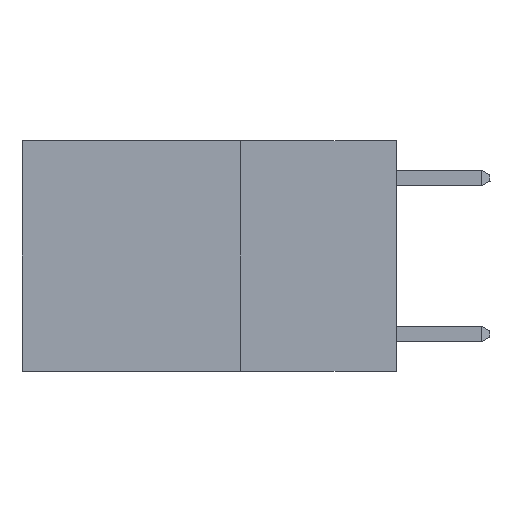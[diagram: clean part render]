
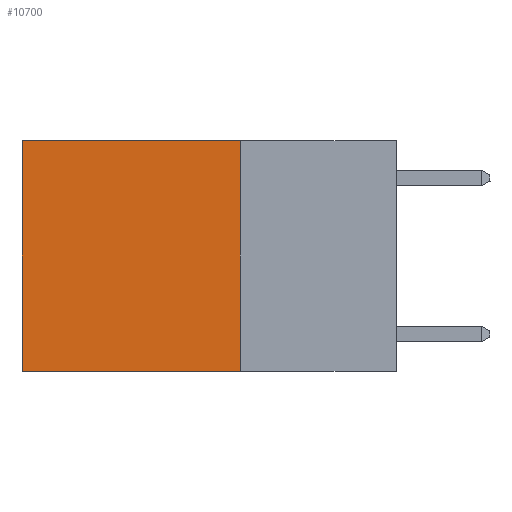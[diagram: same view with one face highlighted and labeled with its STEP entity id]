
A CAD part, left-side view. The second image highlights one B-rep face of the part: STEP entity #10700.
In plain terms, the highlighted planar face has unit normal (-1, 0, 0).
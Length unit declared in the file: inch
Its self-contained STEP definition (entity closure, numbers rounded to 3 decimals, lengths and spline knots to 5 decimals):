
#1501 = VERTEX_POINT ( 'NONE', #17438 ) ;
#1979 = EDGE_CURVE ( 'NONE', #24790, #1501, #23777, .T. ) ;
#2228 = DIRECTION ( 'NONE',  ( 0., 0., -1. ) ) ;
#2391 = VECTOR ( 'NONE', #21699, 39.37008 ) ;
#3250 = ORIENTED_EDGE ( 'NONE', *, *, #13745, .F. ) ;
#4246 = LINE ( 'NONE', #12738, #13555 ) ;
#4757 = CARTESIAN_POINT ( 'NONE',  ( 0.2625, 0.25, -0.37 ) ) ;
#6575 = DIRECTION ( 'NONE',  ( 0., 1., 0. ) ) ;
#9055 = DIRECTION ( 'NONE',  ( 0., 0., -1. ) ) ;
#9156 = VECTOR ( 'NONE', #6575, 39.37008 ) ;
#10002 = EDGE_LOOP ( 'NONE', ( #15845, #26331, #3250, #17077 ) ) ;
#10683 = VECTOR ( 'NONE', #9055, 39.37008 ) ;
#10700 = ADVANCED_FACE ( 'NONE', ( #14855 ), #15138, .F. ) ;
#11227 = CARTESIAN_POINT ( 'NONE',  ( 0.2625, 0.25, -0.37 ) ) ;
#12738 = CARTESIAN_POINT ( 'NONE',  ( 0.2625, 0.25, 0. ) ) ;
#13242 = LINE ( 'NONE', #23913, #10683 ) ;
#13253 = CARTESIAN_POINT ( 'NONE',  ( 0.2625, 0.6, 0. ) ) ;
#13555 = VECTOR ( 'NONE', #25208, 39.37008 ) ;
#13745 = EDGE_CURVE ( 'NONE', #18843, #26649, #13242, .T. ) ;
#14855 = FACE_OUTER_BOUND ( 'NONE', #10002, .T. ) ;
#15138 = PLANE ( 'NONE',  #23408 ) ;
#15565 = CARTESIAN_POINT ( 'NONE',  ( 0.2625, 0.25, 0. ) ) ;
#15845 = ORIENTED_EDGE ( 'NONE', *, *, #1979, .T. ) ;
#17077 = ORIENTED_EDGE ( 'NONE', *, *, #21356, .T. ) ;
#17438 = CARTESIAN_POINT ( 'NONE',  ( 0.2625, 0.6, -0.37 ) ) ;
#18843 = VERTEX_POINT ( 'NONE', #15565 ) ;
#20287 = CARTESIAN_POINT ( 'NONE',  ( 0.2625, 0.6, 0. ) ) ;
#21217 = DIRECTION ( 'NONE',  ( 1., 0., 0. ) ) ;
#21356 = EDGE_CURVE ( 'NONE', #18843, #24790, #4246, .T. ) ;
#21619 = CARTESIAN_POINT ( 'NONE',  ( 0.2625, 0.25, 0. ) ) ;
#21699 = DIRECTION ( 'NONE',  ( 0., 0., -1. ) ) ;
#23408 = AXIS2_PLACEMENT_3D ( 'NONE', #21619, #21217, #2228 ) ;
#23770 = LINE ( 'NONE', #4757, #9156 ) ;
#23777 = LINE ( 'NONE', #13253, #2391 ) ;
#23913 = CARTESIAN_POINT ( 'NONE',  ( 0.2625, 0.25, 0. ) ) ;
#24567 = EDGE_CURVE ( 'NONE', #26649, #1501, #23770, .T. ) ;
#24790 = VERTEX_POINT ( 'NONE', #20287 ) ;
#25208 = DIRECTION ( 'NONE',  ( 0., 1., 0. ) ) ;
#26331 = ORIENTED_EDGE ( 'NONE', *, *, #24567, .F. ) ;
#26649 = VERTEX_POINT ( 'NONE', #11227 ) ;
